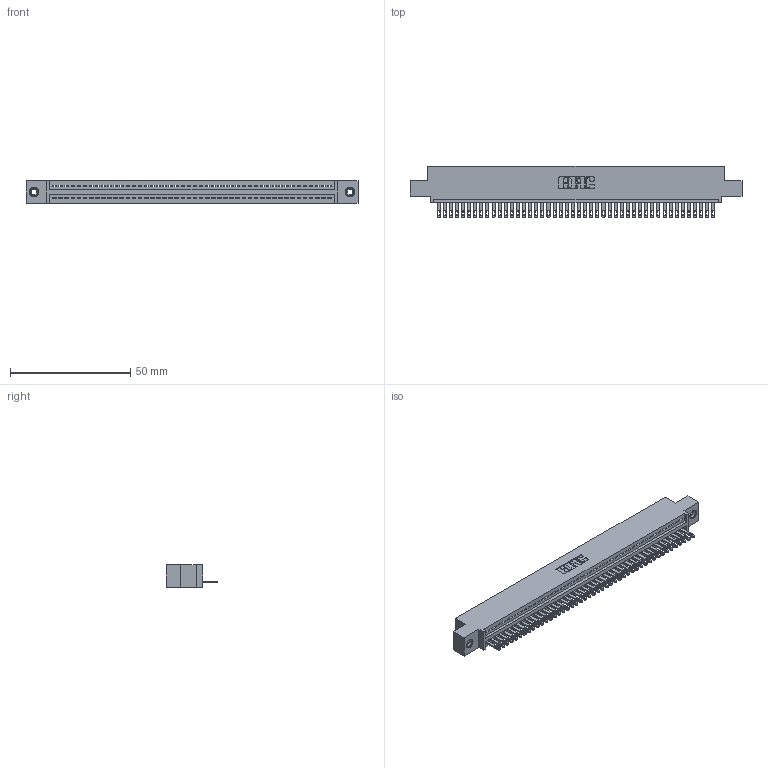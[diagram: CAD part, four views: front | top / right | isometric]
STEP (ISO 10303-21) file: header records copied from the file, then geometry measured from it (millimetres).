
FILE_DESCRIPTION (( 'STEP AP203' ), '1' );
FILE_NAME ('895-046-500-408.STEP', '2020-09-27T04:50:48', ( '' ), ( '' ), 'SwSTEP 2.0', 'SolidWorks 2020', '' );
FILE_SCHEMA (( 'CONFIG_CONTROL_DESIGN' ));
Length unit declared in the file: inch
Products named in the file (4): 345-250-001_345-250-003-102; 895-046-500-408; 345-292-001_345-293-100; 845 Part_0.110 Offset - 0.156 Dia-TI
Assembly tree (49 placements, depth 2):
  895-046-500-408
    845 Part_0.110 Offset - 0.156 Dia-TI
    345-292-001_345-293-100  x46
    345-250-001_345-250-003-102  x2
Bounding box: 138.05 x 21.51 x 9.4 mm (x, y, z)
Volume: 13093.4 mm3; surface area: 17658.6 mm2
Topology: 49 solids, 49 shells, 2674 faces, 8217 edges, 5470 vertices
Faces by surface type: plane 1680, cylinder 978, cone 12, torus 4
Entity records: 35330 total; most frequent: CARTESIAN_POINT 6101, ORIENTED_EDGE 6074, DIRECTION 5351, EDGE_CURVE 3037, VECTOR 2697, LINE 2697, VERTEX_POINT 2020, AXIS2_PLACEMENT_3D 1327
